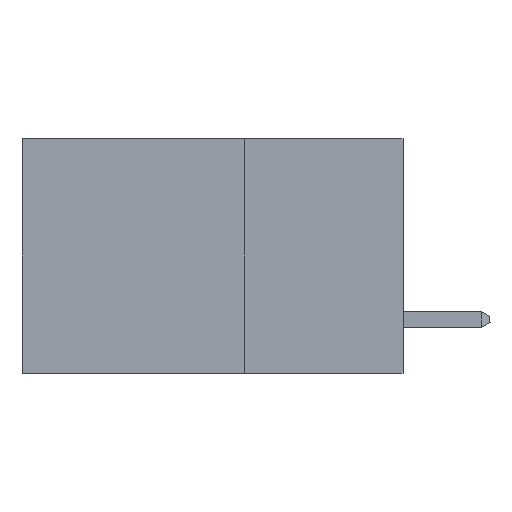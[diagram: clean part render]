
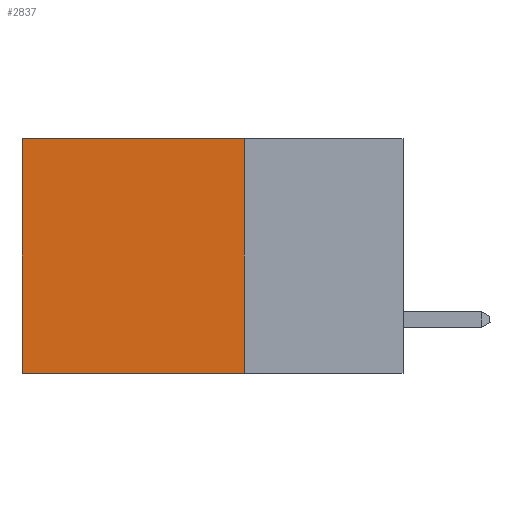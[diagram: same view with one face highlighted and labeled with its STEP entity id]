
A CAD part, left-side view. The second image highlights one B-rep face of the part: STEP entity #2837.
In plain terms, the highlighted planar face has unit normal (-1, 0, 0).
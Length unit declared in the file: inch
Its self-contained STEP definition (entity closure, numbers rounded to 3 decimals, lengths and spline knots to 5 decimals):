
#293 = VECTOR ( 'NONE', #11750, 39.37008 ) ;
#547 = EDGE_LOOP ( 'NONE', ( #13115, #11940, #8927, #10349 ) ) ;
#1675 = DIRECTION ( 'NONE',  ( 0., 0., -1. ) ) ;
#2837 = ADVANCED_FACE ( 'NONE', ( #12713 ), #4785, .F. ) ;
#3090 = DIRECTION ( 'NONE',  ( 0., 0., -1. ) ) ;
#3327 = VERTEX_POINT ( 'NONE', #9567 ) ;
#3385 = CARTESIAN_POINT ( 'NONE',  ( 0.2875, 0.6, -0.37 ) ) ;
#3842 = CARTESIAN_POINT ( 'NONE',  ( 0.2875, 0.25, 0. ) ) ;
#4072 = LINE ( 'NONE', #11946, #9041 ) ;
#4675 = DIRECTION ( 'NONE',  ( 1., 0., 0. ) ) ;
#4785 = PLANE ( 'NONE',  #9027 ) ;
#5121 = CARTESIAN_POINT ( 'NONE',  ( 0.2875, 0.25, 0. ) ) ;
#5159 = CARTESIAN_POINT ( 'NONE',  ( 0.2875, 0.25, -0.37 ) ) ;
#6437 = VECTOR ( 'NONE', #1675, 39.37008 ) ;
#6833 = DIRECTION ( 'NONE',  ( 0., 0., -1. ) ) ;
#8163 = LINE ( 'NONE', #5159, #12323 ) ;
#8235 = CARTESIAN_POINT ( 'NONE',  ( 0.2875, 0.6, 0. ) ) ;
#8927 = ORIENTED_EDGE ( 'NONE', *, *, #13326, .F. ) ;
#9027 = AXIS2_PLACEMENT_3D ( 'NONE', #3842, #4675, #6833 ) ;
#9041 = VECTOR ( 'NONE', #3090, 39.37008 ) ;
#9544 = CARTESIAN_POINT ( 'NONE',  ( 0.2875, 0.25, -0.37 ) ) ;
#9567 = CARTESIAN_POINT ( 'NONE',  ( 0.2875, 0.6, 0. ) ) ;
#9595 = DIRECTION ( 'NONE',  ( 0., 1., 0. ) ) ;
#9825 = EDGE_CURVE ( 'NONE', #3327, #13535, #13574, .T. ) ;
#10089 = LINE ( 'NONE', #10644, #293 ) ;
#10349 = ORIENTED_EDGE ( 'NONE', *, *, #13348, .T. ) ;
#10644 = CARTESIAN_POINT ( 'NONE',  ( 0.2875, 0.25, 0. ) ) ;
#11423 = VERTEX_POINT ( 'NONE', #9544 ) ;
#11750 = DIRECTION ( 'NONE',  ( 0., 1., 0. ) ) ;
#11940 = ORIENTED_EDGE ( 'NONE', *, *, #14109, .F. ) ;
#11946 = CARTESIAN_POINT ( 'NONE',  ( 0.2875, 0.25, 0. ) ) ;
#12323 = VECTOR ( 'NONE', #9595, 39.37008 ) ;
#12681 = VERTEX_POINT ( 'NONE', #5121 ) ;
#12713 = FACE_OUTER_BOUND ( 'NONE', #547, .T. ) ;
#13115 = ORIENTED_EDGE ( 'NONE', *, *, #9825, .T. ) ;
#13326 = EDGE_CURVE ( 'NONE', #12681, #11423, #4072, .T. ) ;
#13348 = EDGE_CURVE ( 'NONE', #12681, #3327, #10089, .T. ) ;
#13535 = VERTEX_POINT ( 'NONE', #3385 ) ;
#13574 = LINE ( 'NONE', #8235, #6437 ) ;
#14109 = EDGE_CURVE ( 'NONE', #11423, #13535, #8163, .T. ) ;
